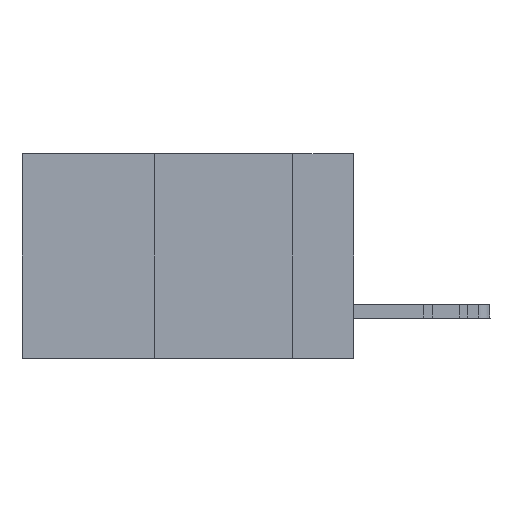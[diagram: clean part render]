
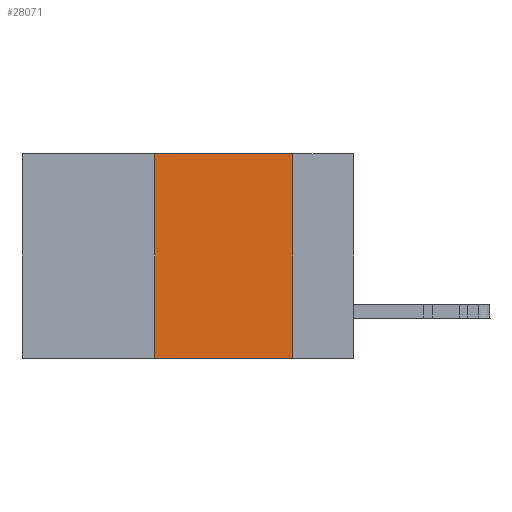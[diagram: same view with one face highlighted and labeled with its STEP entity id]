
A CAD part, left-side view. The second image highlights one B-rep face of the part: STEP entity #28071.
In plain terms, the highlighted planar face has unit normal (-1, 0, 0).
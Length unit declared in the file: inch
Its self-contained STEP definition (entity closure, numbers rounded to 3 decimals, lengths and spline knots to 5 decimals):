
#291 = VECTOR ( 'NONE', #22990, 39.37008 ) ;
#1392 = EDGE_CURVE ( 'NONE', #3118, #40098, #27447, .T. ) ;
#3118 = VERTEX_POINT ( 'NONE', #16449 ) ;
#4678 = DIRECTION ( 'NONE',  ( 1., 0., 0. ) ) ;
#6453 = EDGE_CURVE ( 'NONE', #29919, #15606, #26336, .T. ) ;
#8660 = DIRECTION ( 'NONE',  ( 0., 0., -1. ) ) ;
#9854 = VECTOR ( 'NONE', #39716, 39.37008 ) ;
#10021 = ORIENTED_EDGE ( 'NONE', *, *, #32076, .F. ) ;
#11525 = CARTESIAN_POINT ( 'NONE',  ( 0., 0.11, 0. ) ) ;
#15606 = VERTEX_POINT ( 'NONE', #27785 ) ;
#16449 = CARTESIAN_POINT ( 'NONE',  ( 0., 0.36, 0. ) ) ;
#17073 = ORIENTED_EDGE ( 'NONE', *, *, #6453, .T. ) ;
#17776 = VECTOR ( 'NONE', #32650, 39.37008 ) ;
#18208 = PLANE ( 'NONE',  #37629 ) ;
#19116 = EDGE_CURVE ( 'NONE', #29919, #3118, #40669, .T. ) ;
#20651 = CARTESIAN_POINT ( 'NONE',  ( 0., 0.6, 0. ) ) ;
#22990 = DIRECTION ( 'NONE',  ( 0., -1., 0. ) ) ;
#25032 = CARTESIAN_POINT ( 'NONE',  ( 0., 0.6, 0. ) ) ;
#25671 = CARTESIAN_POINT ( 'NONE',  ( 0., 0.36, 0. ) ) ;
#25813 = FACE_OUTER_BOUND ( 'NONE', #35518, .T. ) ;
#26336 = LINE ( 'NONE', #26705, #291 ) ;
#26705 = CARTESIAN_POINT ( 'NONE',  ( 0., 0.6, -0.37 ) ) ;
#27447 = LINE ( 'NONE', #20651, #9854 ) ;
#27785 = CARTESIAN_POINT ( 'NONE',  ( 0., 0.11, -0.37 ) ) ;
#28071 = ADVANCED_FACE ( 'NONE', ( #25813 ), #18208, .F. ) ;
#28807 = CARTESIAN_POINT ( 'NONE',  ( 0., 0.11, 0. ) ) ;
#29919 = VERTEX_POINT ( 'NONE', #36973 ) ;
#30964 = ORIENTED_EDGE ( 'NONE', *, *, #1392, .F. ) ;
#32076 = EDGE_CURVE ( 'NONE', #40098, #15606, #37275, .T. ) ;
#32650 = DIRECTION ( 'NONE',  ( 0., 0., 1. ) ) ;
#35518 = EDGE_LOOP ( 'NONE', ( #10021, #30964, #37547, #17073 ) ) ;
#36973 = CARTESIAN_POINT ( 'NONE',  ( 0., 0.36, -0.37 ) ) ;
#37275 = LINE ( 'NONE', #11525, #38325 ) ;
#37547 = ORIENTED_EDGE ( 'NONE', *, *, #19116, .F. ) ;
#37629 = AXIS2_PLACEMENT_3D ( 'NONE', #25032, #4678, #39446 ) ;
#38325 = VECTOR ( 'NONE', #8660, 39.37008 ) ;
#39446 = DIRECTION ( 'NONE',  ( 0., 0., -1. ) ) ;
#39716 = DIRECTION ( 'NONE',  ( 0., -1., 0. ) ) ;
#40098 = VERTEX_POINT ( 'NONE', #28807 ) ;
#40669 = LINE ( 'NONE', #25671, #17776 ) ;
